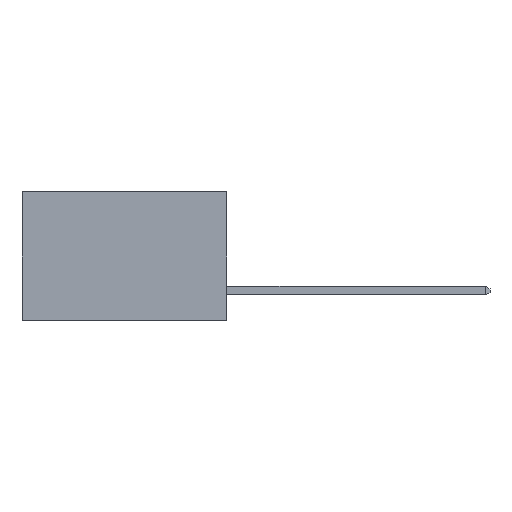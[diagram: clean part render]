
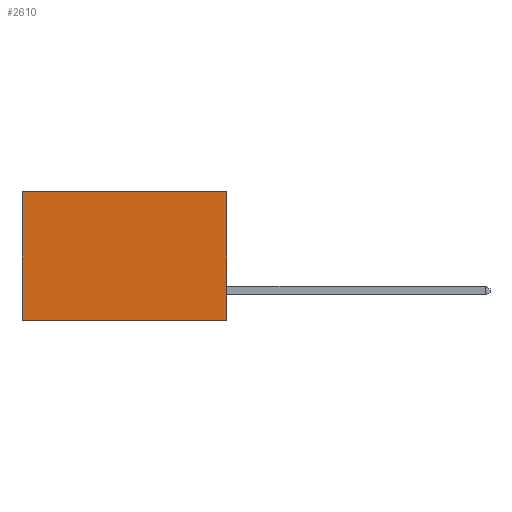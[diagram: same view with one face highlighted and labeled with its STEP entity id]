
A CAD part, left-side view. The second image highlights one B-rep face of the part: STEP entity #2610.
In plain terms, the highlighted planar face has unit normal (-1, 0, 0).
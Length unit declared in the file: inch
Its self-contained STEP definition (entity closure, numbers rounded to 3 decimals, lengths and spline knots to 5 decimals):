
#433 = DIRECTION ( 'NONE',  ( 1., 0., 0. ) ) ;
#435 = ORIENTED_EDGE ( 'NONE', *, *, #5838, .F. ) ;
#767 = LINE ( 'NONE', #4583, #2566 ) ;
#902 = VERTEX_POINT ( 'NONE', #8936 ) ;
#1559 = DIRECTION ( 'NONE',  ( 0., 1., 0. ) ) ;
#1906 = EDGE_LOOP ( 'NONE', ( #8125, #435, #4541, #5310 ) ) ;
#2451 = CARTESIAN_POINT ( 'NONE',  ( 0.277, 0., -0.37 ) ) ;
#2495 = DIRECTION ( 'NONE',  ( 0., 1., 0. ) ) ;
#2566 = VECTOR ( 'NONE', #4313, 39.37008 ) ;
#2610 = ADVANCED_FACE ( 'NONE', ( #2977 ), #5546, .F. ) ;
#2977 = FACE_OUTER_BOUND ( 'NONE', #1906, .T. ) ;
#3015 = EDGE_CURVE ( 'NONE', #9024, #4809, #5949, .T. ) ;
#3057 = CARTESIAN_POINT ( 'NONE',  ( 0.277, 0.59, 0. ) ) ;
#3685 = CARTESIAN_POINT ( 'NONE',  ( 0.277, 0., -0.37 ) ) ;
#3729 = AXIS2_PLACEMENT_3D ( 'NONE', #3685, #433, #4765 ) ;
#4189 = VECTOR ( 'NONE', #1559, 39.37008 ) ;
#4313 = DIRECTION ( 'NONE',  ( 0., 0., -1. ) ) ;
#4541 = ORIENTED_EDGE ( 'NONE', *, *, #6265, .F. ) ;
#4583 = CARTESIAN_POINT ( 'NONE',  ( 0.277, 0., -0.37 ) ) ;
#4701 = CARTESIAN_POINT ( 'NONE',  ( 0.277, 0., 0. ) ) ;
#4765 = DIRECTION ( 'NONE',  ( 0., 0., -1. ) ) ;
#4809 = VERTEX_POINT ( 'NONE', #3057 ) ;
#5310 = ORIENTED_EDGE ( 'NONE', *, *, #3015, .T. ) ;
#5546 = PLANE ( 'NONE',  #3729 ) ;
#5761 = VECTOR ( 'NONE', #7174, 39.37008 ) ;
#5838 = EDGE_CURVE ( 'NONE', #902, #6741, #8241, .T. ) ;
#5949 = LINE ( 'NONE', #4701, #4189 ) ;
#5990 = LINE ( 'NONE', #6657, #5761 ) ;
#6265 = EDGE_CURVE ( 'NONE', #9024, #902, #767, .T. ) ;
#6657 = CARTESIAN_POINT ( 'NONE',  ( 0.277, 0.59, -0.37 ) ) ;
#6741 = VERTEX_POINT ( 'NONE', #7603 ) ;
#6942 = CARTESIAN_POINT ( 'NONE',  ( 0.277, 0., 0. ) ) ;
#7174 = DIRECTION ( 'NONE',  ( 0., 0., -1. ) ) ;
#7603 = CARTESIAN_POINT ( 'NONE',  ( 0.277, 0.59, -0.37 ) ) ;
#8027 = VECTOR ( 'NONE', #2495, 39.37008 ) ;
#8125 = ORIENTED_EDGE ( 'NONE', *, *, #9172, .T. ) ;
#8241 = LINE ( 'NONE', #2451, #8027 ) ;
#8936 = CARTESIAN_POINT ( 'NONE',  ( 0.277, 0., -0.37 ) ) ;
#9024 = VERTEX_POINT ( 'NONE', #6942 ) ;
#9172 = EDGE_CURVE ( 'NONE', #4809, #6741, #5990, .T. ) ;
